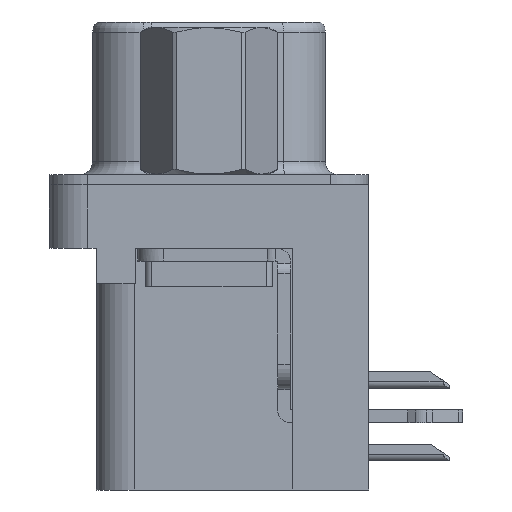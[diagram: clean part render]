
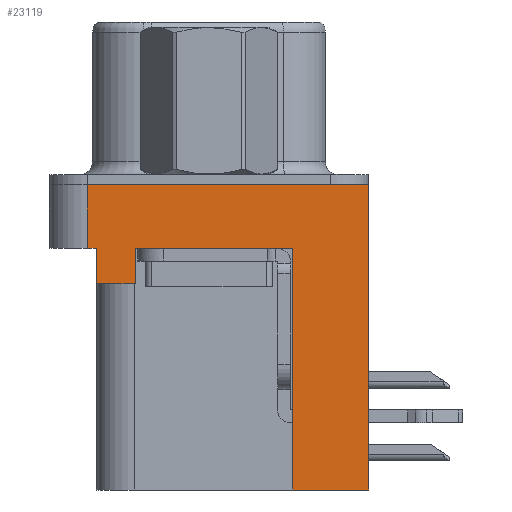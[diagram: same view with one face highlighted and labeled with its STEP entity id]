
A CAD part, left-side view. The second image highlights one B-rep face of the part: STEP entity #23119.
In plain terms, the highlighted planar face has unit normal (-1, 0, 0).
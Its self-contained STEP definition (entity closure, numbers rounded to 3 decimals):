
#316 = CARTESIAN_POINT ( 'NONE',  ( -2.935, -3.295, -2.5 ) ) ;
#377 = VECTOR ( 'NONE', #20775, 1000. ) ;
#1207 = PLANE ( 'NONE',  #13587 ) ;
#1290 = EDGE_CURVE ( 'NONE', #11279, #17935, #9295, .T. ) ;
#2030 = VECTOR ( 'NONE', #20736, 1000. ) ;
#2406 = VERTEX_POINT ( 'NONE', #316 ) ;
#2412 = DIRECTION ( 'NONE',  ( 0., 0., 1. ) ) ;
#3535 = VERTEX_POINT ( 'NONE', #23766 ) ;
#4548 = CARTESIAN_POINT ( 'NONE',  ( -2.935, -6.275, -2.5 ) ) ;
#4553 = CARTESIAN_POINT ( 'NONE',  ( -2.935, -6.275, 0. ) ) ;
#4559 = CARTESIAN_POINT ( 'NONE',  ( -2.935, 4.425, -2.5 ) ) ;
#4612 = CARTESIAN_POINT ( 'NONE',  ( -2.935, 4.775, -2.5 ) ) ;
#4636 = ORIENTED_EDGE ( 'NONE', *, *, #1290, .T. ) ;
#5077 = CARTESIAN_POINT ( 'NONE',  ( -2.935, 4.425, -3.9 ) ) ;
#5426 = ORIENTED_EDGE ( 'NONE', *, *, #14580, .F. ) ;
#5527 = CARTESIAN_POINT ( 'NONE',  ( -2.935, 4.425, -3.9 ) ) ;
#6044 = ORIENTED_EDGE ( 'NONE', *, *, #18606, .T. ) ;
#6130 = ORIENTED_EDGE ( 'NONE', *, *, #10364, .F. ) ;
#6214 = DIRECTION ( 'NONE',  ( 0., 0., 1. ) ) ;
#6834 = EDGE_CURVE ( 'NONE', #17253, #8022, #21615, .T. ) ;
#6944 = CARTESIAN_POINT ( 'NONE',  ( -2.935, 2.895, -3.9 ) ) ;
#7122 = CARTESIAN_POINT ( 'NONE',  ( -2.935, 4.775, -2.5 ) ) ;
#7367 = DIRECTION ( 'NONE',  ( 0., 1., 0. ) ) ;
#7626 = LINE ( 'NONE', #4612, #18829 ) ;
#7778 = ORIENTED_EDGE ( 'NONE', *, *, #6834, .F. ) ;
#7809 = ORIENTED_EDGE ( 'NONE', *, *, #8286, .T. ) ;
#8022 = VERTEX_POINT ( 'NONE', #4559 ) ;
#8038 = CARTESIAN_POINT ( 'NONE',  ( -2.935, -6.275, -2.5 ) ) ;
#8041 = LINE ( 'NONE', #4548, #23624 ) ;
#8286 = EDGE_CURVE ( 'NONE', #12796, #8022, #20356, .T. ) ;
#8421 = EDGE_CURVE ( 'NONE', #9123, #2406, #12708, .T. ) ;
#8649 = CARTESIAN_POINT ( 'NONE',  ( -2.935, -6.275, -12. ) ) ;
#8803 = CARTESIAN_POINT ( 'NONE',  ( -2.935, -3.295, -12. ) ) ;
#9123 = VERTEX_POINT ( 'NONE', #8803 ) ;
#9295 = LINE ( 'NONE', #9512, #23687 ) ;
#9512 = CARTESIAN_POINT ( 'NONE',  ( -2.935, 2.895, -3.9 ) ) ;
#10036 = EDGE_LOOP ( 'NONE', ( #21571, #6130, #7809, #7778, #5426, #4636, #6044, #15208, #18571, #13269 ) ) ;
#10178 = EDGE_CURVE ( 'NONE', #18423, #3535, #23223, .T. ) ;
#10364 = EDGE_CURVE ( 'NONE', #12796, #18423, #7626, .T. ) ;
#11279 = VERTEX_POINT ( 'NONE', #6944 ) ;
#11809 = DIRECTION ( 'NONE',  ( 0., -1., 0. ) ) ;
#12428 = VECTOR ( 'NONE', #7367, 1000. ) ;
#12656 = VECTOR ( 'NONE', #17128, 1000. ) ;
#12708 = LINE ( 'NONE', #15205, #2030 ) ;
#12796 = VERTEX_POINT ( 'NONE', #7122 ) ;
#13269 = ORIENTED_EDGE ( 'NONE', *, *, #16165, .T. ) ;
#13301 = CARTESIAN_POINT ( 'NONE',  ( -2.935, -6.275, -2.5 ) ) ;
#13587 = AXIS2_PLACEMENT_3D ( 'NONE', #23975, #16169, #20123 ) ;
#14185 = DIRECTION ( 'NONE',  ( 0., 0., 1. ) ) ;
#14580 = EDGE_CURVE ( 'NONE', #11279, #17253, #15472, .T. ) ;
#15205 = CARTESIAN_POINT ( 'NONE',  ( -2.935, -3.295, -12. ) ) ;
#15208 = ORIENTED_EDGE ( 'NONE', *, *, #8421, .F. ) ;
#15253 = VERTEX_POINT ( 'NONE', #8649 ) ;
#15472 = LINE ( 'NONE', #5527, #377 ) ;
#16005 = DIRECTION ( 'NONE',  ( 0., -1., 0. ) ) ;
#16165 = EDGE_CURVE ( 'NONE', #15253, #3535, #8041, .T. ) ;
#16169 = DIRECTION ( 'NONE',  ( -1., 0., 0. ) ) ;
#17128 = DIRECTION ( 'NONE',  ( 0., -1., 0. ) ) ;
#17253 = VERTEX_POINT ( 'NONE', #5077 ) ;
#17366 = EDGE_CURVE ( 'NONE', #15253, #9123, #17399, .T. ) ;
#17399 = LINE ( 'NONE', #18731, #12428 ) ;
#17935 = VERTEX_POINT ( 'NONE', #19235 ) ;
#18235 = VECTOR ( 'NONE', #16005, 1000. ) ;
#18423 = VERTEX_POINT ( 'NONE', #22423 ) ;
#18571 = ORIENTED_EDGE ( 'NONE', *, *, #17366, .F. ) ;
#18606 = EDGE_CURVE ( 'NONE', #17935, #2406, #24400, .T. ) ;
#18731 = CARTESIAN_POINT ( 'NONE',  ( -2.935, -3.295, -12. ) ) ;
#18829 = VECTOR ( 'NONE', #14185, 1000. ) ;
#19167 = VECTOR ( 'NONE', #11809, 1000. ) ;
#19235 = CARTESIAN_POINT ( 'NONE',  ( -2.935, 2.895, -2.5 ) ) ;
#19866 = FACE_OUTER_BOUND ( 'NONE', #10036, .T. ) ;
#20123 = DIRECTION ( 'NONE',  ( 0., 0., 1. ) ) ;
#20356 = LINE ( 'NONE', #8038, #19167 ) ;
#20736 = DIRECTION ( 'NONE',  ( 0., 0., 1. ) ) ;
#20775 = DIRECTION ( 'NONE',  ( 0., 1., 0. ) ) ;
#21571 = ORIENTED_EDGE ( 'NONE', *, *, #10178, .F. ) ;
#21615 = LINE ( 'NONE', #22792, #24227 ) ;
#22423 = CARTESIAN_POINT ( 'NONE',  ( -2.935, 4.775, 0. ) ) ;
#22669 = DIRECTION ( 'NONE',  ( 0., 0., 1. ) ) ;
#22792 = CARTESIAN_POINT ( 'NONE',  ( -2.935, 4.425, -3.9 ) ) ;
#23119 = ADVANCED_FACE ( 'NONE', ( #19866 ), #1207, .T. ) ;
#23223 = LINE ( 'NONE', #4553, #18235 ) ;
#23624 = VECTOR ( 'NONE', #6214, 1000. ) ;
#23687 = VECTOR ( 'NONE', #22669, 1000. ) ;
#23766 = CARTESIAN_POINT ( 'NONE',  ( -2.935, -6.275, 0. ) ) ;
#23975 = CARTESIAN_POINT ( 'NONE',  ( -2.935, -6.275, -2.5 ) ) ;
#24227 = VECTOR ( 'NONE', #2412, 1000. ) ;
#24400 = LINE ( 'NONE', #13301, #12656 ) ;
